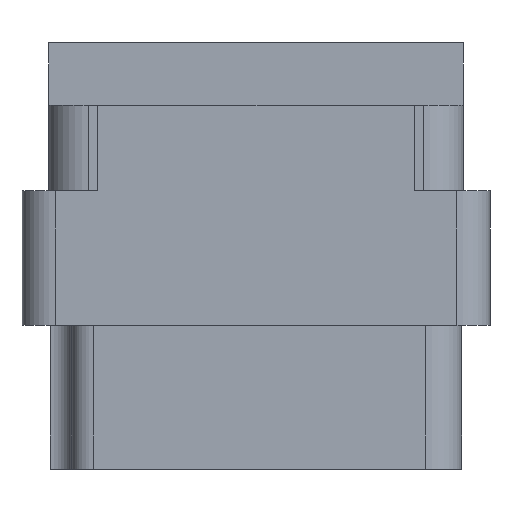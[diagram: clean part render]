
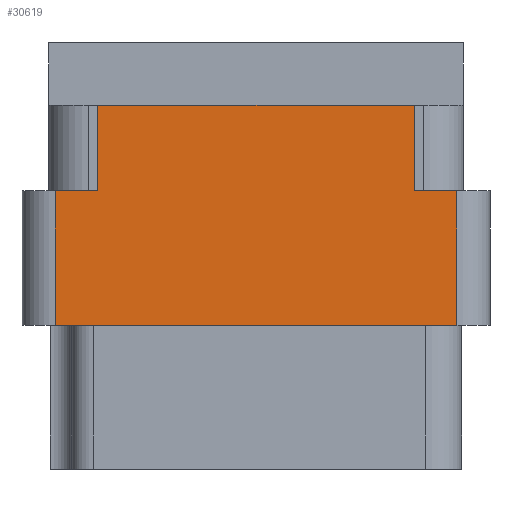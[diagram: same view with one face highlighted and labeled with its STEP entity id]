
A CAD part, left-side view. The second image highlights one B-rep face of the part: STEP entity #30619.
In plain terms, the highlighted planar face has unit normal (-1, 0, 0).
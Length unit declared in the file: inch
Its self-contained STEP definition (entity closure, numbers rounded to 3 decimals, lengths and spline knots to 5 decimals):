
#199 = EDGE_CURVE ( 'NONE', #22169, #8973, #16798, .T. ) ;
#452 = VERTEX_POINT ( 'NONE', #28974 ) ;
#1870 = LINE ( 'NONE', #38345, #22439 ) ;
#2042 = VECTOR ( 'NONE', #24166, 39.37008 ) ;
#2640 = DIRECTION ( 'NONE',  ( 0., 0., 1. ) ) ;
#3675 = VECTOR ( 'NONE', #2640, 39.37008 ) ;
#5110 = DIRECTION ( 'NONE',  ( -1., 0., 0. ) ) ;
#7747 = DIRECTION ( 'NONE',  ( 0., 0., 1. ) ) ;
#8273 = ORIENTED_EDGE ( 'NONE', *, *, #17520, .T. ) ;
#8306 = VERTEX_POINT ( 'NONE', #25058 ) ;
#8896 = EDGE_CURVE ( 'NONE', #24597, #9173, #25690, .T. ) ;
#8973 = VERTEX_POINT ( 'NONE', #20083 ) ;
#9173 = VERTEX_POINT ( 'NONE', #42256 ) ;
#9421 = ORIENTED_EDGE ( 'NONE', *, *, #41380, .F. ) ;
#9582 = ORIENTED_EDGE ( 'NONE', *, *, #8896, .F. ) ;
#10086 = ORIENTED_EDGE ( 'NONE', *, *, #24601, .T. ) ;
#10395 = VERTEX_POINT ( 'NONE', #24307 ) ;
#10715 = EDGE_LOOP ( 'NONE', ( #19089, #8273, #9582, #22864, #21069, #10086, #38423, #9421 ) ) ;
#11206 = CARTESIAN_POINT ( 'NONE',  ( -1.296, 0.296, -0.277 ) ) ;
#11478 = CARTESIAN_POINT ( 'NONE',  ( -1.296, -0.376, -0.277 ) ) ;
#12550 = CARTESIAN_POINT ( 'NONE',  ( -1.296, -0.376, -0.798 ) ) ;
#15029 = AXIS2_PLACEMENT_3D ( 'NONE', #34892, #5110, #31865 ) ;
#15059 = VECTOR ( 'NONE', #31034, 39.37008 ) ;
#15277 = DIRECTION ( 'NONE',  ( 0., -1., 0. ) ) ;
#16798 = LINE ( 'NONE', #40844, #39009 ) ;
#17513 = CARTESIAN_POINT ( 'NONE',  ( -1.296, -0.376, -0.529 ) ) ;
#17520 = EDGE_CURVE ( 'NONE', #8306, #9173, #19343, .T. ) ;
#17811 = LINE ( 'NONE', #11206, #27030 ) ;
#19089 = ORIENTED_EDGE ( 'NONE', *, *, #42642, .F. ) ;
#19343 = LINE ( 'NONE', #21032, #27032 ) ;
#20066 = VECTOR ( 'NONE', #42291, 39.37008 ) ;
#20083 = CARTESIAN_POINT ( 'NONE',  ( -1.296, -0.296, -0.117 ) ) ;
#20959 = CARTESIAN_POINT ( 'NONE',  ( -1.296, -0.296, -0.277 ) ) ;
#21032 = CARTESIAN_POINT ( 'NONE',  ( -1.296, 0.376, -0.798 ) ) ;
#21069 = ORIENTED_EDGE ( 'NONE', *, *, #38674, .F. ) ;
#22169 = VERTEX_POINT ( 'NONE', #41135 ) ;
#22439 = VECTOR ( 'NONE', #15277, 39.37008 ) ;
#22864 = ORIENTED_EDGE ( 'NONE', *, *, #25092, .T. ) ;
#24166 = DIRECTION ( 'NONE',  ( 0., -1., 0. ) ) ;
#24307 = CARTESIAN_POINT ( 'NONE',  ( -1.296, 0.296, -0.277 ) ) ;
#24597 = VERTEX_POINT ( 'NONE', #17513 ) ;
#24601 = EDGE_CURVE ( 'NONE', #452, #8973, #37208, .T. ) ;
#25058 = CARTESIAN_POINT ( 'NONE',  ( -1.296, 0.376, -0.277 ) ) ;
#25092 = EDGE_CURVE ( 'NONE', #24597, #31317, #33553, .T. ) ;
#25690 = LINE ( 'NONE', #35943, #20066 ) ;
#27030 = VECTOR ( 'NONE', #7747, 39.37008 ) ;
#27032 = VECTOR ( 'NONE', #27495, 39.37008 ) ;
#27495 = DIRECTION ( 'NONE',  ( 0., 0., -1. ) ) ;
#27545 = DIRECTION ( 'NONE',  ( 0., -1., 0. ) ) ;
#27691 = FACE_OUTER_BOUND ( 'NONE', #10715, .T. ) ;
#28974 = CARTESIAN_POINT ( 'NONE',  ( -1.296, -0.296, -0.277 ) ) ;
#30619 = ADVANCED_FACE ( 'NONE', ( #27691 ), #38367, .T. ) ;
#31034 = DIRECTION ( 'NONE',  ( 0., 0., 1. ) ) ;
#31317 = VERTEX_POINT ( 'NONE', #11478 ) ;
#31377 = LINE ( 'NONE', #40495, #2042 ) ;
#31865 = DIRECTION ( 'NONE',  ( 0., 0., 1. ) ) ;
#33553 = LINE ( 'NONE', #12550, #3675 ) ;
#34892 = CARTESIAN_POINT ( 'NONE',  ( -1.296, -0.438, -0.798 ) ) ;
#35943 = CARTESIAN_POINT ( 'NONE',  ( -1.296, 0., -0.529 ) ) ;
#37208 = LINE ( 'NONE', #20959, #15059 ) ;
#38345 = CARTESIAN_POINT ( 'NONE',  ( -1.296, 0., -0.277 ) ) ;
#38367 = PLANE ( 'NONE',  #15029 ) ;
#38423 = ORIENTED_EDGE ( 'NONE', *, *, #199, .F. ) ;
#38674 = EDGE_CURVE ( 'NONE', #452, #31317, #31377, .T. ) ;
#39009 = VECTOR ( 'NONE', #27545, 39.37008 ) ;
#40495 = CARTESIAN_POINT ( 'NONE',  ( -1.296, 0., -0.277 ) ) ;
#40844 = CARTESIAN_POINT ( 'NONE',  ( -1.296, 0.438, -0.117 ) ) ;
#41135 = CARTESIAN_POINT ( 'NONE',  ( -1.296, 0.296, -0.117 ) ) ;
#41380 = EDGE_CURVE ( 'NONE', #10395, #22169, #17811, .T. ) ;
#42256 = CARTESIAN_POINT ( 'NONE',  ( -1.296, 0.376, -0.529 ) ) ;
#42291 = DIRECTION ( 'NONE',  ( 0., 1., 0. ) ) ;
#42642 = EDGE_CURVE ( 'NONE', #8306, #10395, #1870, .T. ) ;
